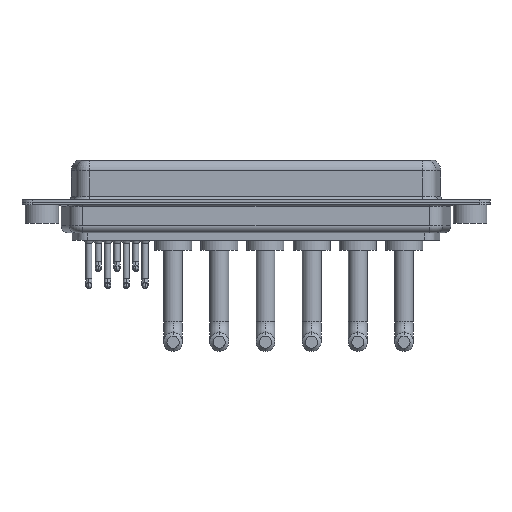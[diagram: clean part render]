
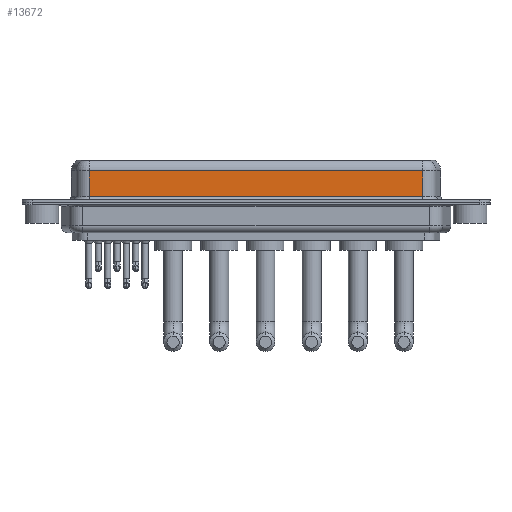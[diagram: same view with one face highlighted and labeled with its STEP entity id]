
A CAD part, front view. The second image highlights one B-rep face of the part: STEP entity #13672.
In plain terms, the highlighted planar face has unit normal (0, -1, 0).
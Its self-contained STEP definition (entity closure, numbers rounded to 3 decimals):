
#56 = LINE ( 'NONE', #12661, #735 ) ;
#100 = CARTESIAN_POINT ( 'NONE',  ( 56.462, -3.95, 0.9 ) ) ;
#125 = ORIENTED_EDGE ( 'NONE', *, *, #9752, .T. ) ;
#735 = VECTOR ( 'NONE', #7063, 1000. ) ;
#1423 = VECTOR ( 'NONE', #10093, 1000. ) ;
#2094 = VECTOR ( 'NONE', #18196, 1000. ) ;
#2724 = CARTESIAN_POINT ( 'NONE',  ( 56.462, -3.95, 4.65 ) ) ;
#3439 = VERTEX_POINT ( 'NONE', #2724 ) ;
#3727 = VERTEX_POINT ( 'NONE', #4961 ) ;
#4253 = ORIENTED_EDGE ( 'NONE', *, *, #16026, .T. ) ;
#4608 = CARTESIAN_POINT ( 'NONE',  ( 56.462, -3.95, 6.4 ) ) ;
#4961 = CARTESIAN_POINT ( 'NONE',  ( 56.462, -3.95, 0.9 ) ) ;
#5047 = DIRECTION ( 'NONE',  ( 0., 1., 0. ) ) ;
#5400 = CARTESIAN_POINT ( 'NONE',  ( 56.462, -3.95, 4.65 ) ) ;
#6628 = FACE_OUTER_BOUND ( 'NONE', #8060, .T. ) ;
#7063 = DIRECTION ( 'NONE',  ( 0., 0., -1. ) ) ;
#7735 = ORIENTED_EDGE ( 'NONE', *, *, #17987, .F. ) ;
#7942 = AXIS2_PLACEMENT_3D ( 'NONE', #4608, #5047, #15134 ) ;
#8060 = EDGE_LOOP ( 'NONE', ( #7735, #9466, #4253, #125 ) ) ;
#8274 = LINE ( 'NONE', #13782, #2094 ) ;
#8344 = VERTEX_POINT ( 'NONE', #15851 ) ;
#9466 = ORIENTED_EDGE ( 'NONE', *, *, #11481, .T. ) ;
#9752 = EDGE_CURVE ( 'NONE', #8344, #3727, #14293, .T. ) ;
#10093 = DIRECTION ( 'NONE',  ( 1., 0., 0. ) ) ;
#11481 = EDGE_CURVE ( 'NONE', #3439, #18365, #18309, .T. ) ;
#12661 = CARTESIAN_POINT ( 'NONE',  ( 56.462, -3.95, 6.4 ) ) ;
#13672 = ADVANCED_FACE ( 'NONE', ( #6628 ), #15225, .F. ) ;
#13782 = CARTESIAN_POINT ( 'NONE',  ( 7.038, -3.95, 6.4 ) ) ;
#14007 = DIRECTION ( 'NONE',  ( -1., 0., 0. ) ) ;
#14293 = LINE ( 'NONE', #100, #1423 ) ;
#15134 = DIRECTION ( 'NONE',  ( 0., 0., 1. ) ) ;
#15225 = PLANE ( 'NONE',  #7942 ) ;
#15851 = CARTESIAN_POINT ( 'NONE',  ( 7.038, -3.95, 0.9 ) ) ;
#16026 = EDGE_CURVE ( 'NONE', #18365, #8344, #8274, .T. ) ;
#16296 = CARTESIAN_POINT ( 'NONE',  ( 7.038, -3.95, 4.65 ) ) ;
#16578 = VECTOR ( 'NONE', #14007, 1000. ) ;
#17987 = EDGE_CURVE ( 'NONE', #3439, #3727, #56, .T. ) ;
#18196 = DIRECTION ( 'NONE',  ( 0., 0., -1. ) ) ;
#18309 = LINE ( 'NONE', #5400, #16578 ) ;
#18365 = VERTEX_POINT ( 'NONE', #16296 ) ;
